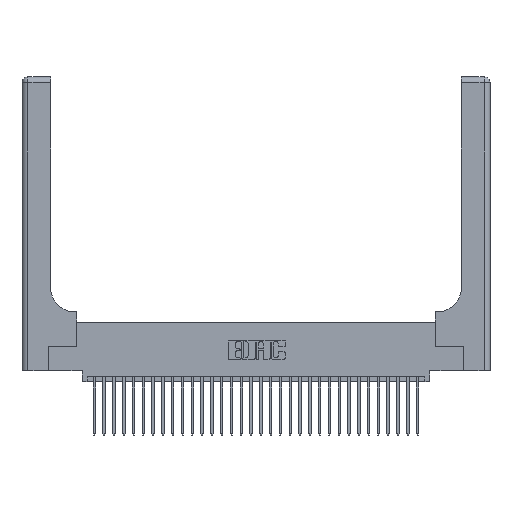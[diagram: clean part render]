
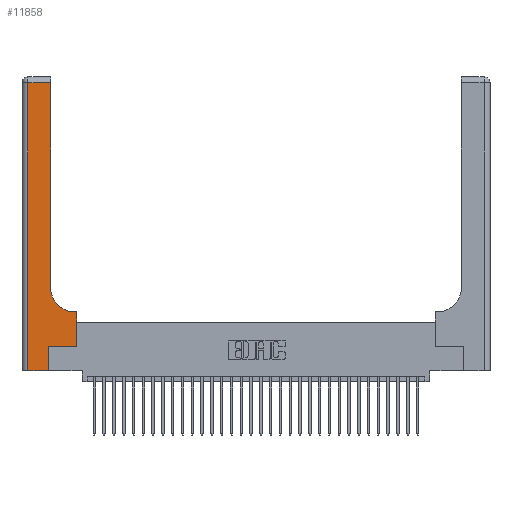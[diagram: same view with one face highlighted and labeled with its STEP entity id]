
A CAD part, top view. The second image highlights one B-rep face of the part: STEP entity #11858.
In plain terms, the highlighted planar face has unit normal (0, 0, 1).
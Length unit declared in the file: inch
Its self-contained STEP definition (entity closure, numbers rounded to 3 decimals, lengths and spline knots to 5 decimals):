
#128 = VECTOR ( 'NONE', #6298, 39.37008 ) ;
#644 = EDGE_CURVE ( 'NONE', #1270, #31202, #12621, .T. ) ;
#1270 = VERTEX_POINT ( 'NONE', #6350 ) ;
#1298 = DIRECTION ( 'NONE',  ( 0., 0., -1. ) ) ;
#2221 = VERTEX_POINT ( 'NONE', #28364 ) ;
#2227 = VERTEX_POINT ( 'NONE', #18069 ) ;
#2339 = EDGE_CURVE ( 'NONE', #2227, #22866, #31743, .T. ) ;
#2566 = EDGE_CURVE ( 'NONE', #31202, #2221, #10892, .T. ) ;
#2685 = EDGE_CURVE ( 'NONE', #2221, #3095, #14499, .T. ) ;
#3095 = VERTEX_POINT ( 'NONE', #18068 ) ;
#3262 = CARTESIAN_POINT ( 'NONE',  ( 0.5415, 0.85, 0.37 ) ) ;
#3271 = VECTOR ( 'NONE', #5865, 39.37008 ) ;
#3285 = CARTESIAN_POINT ( 'NONE',  ( 0.2915, 3., 0.37 ) ) ;
#3651 = LINE ( 'NONE', #20341, #30130 ) ;
#3737 = CARTESIAN_POINT ( 'NONE',  ( 0., 2.94, 0.37 ) ) ;
#3854 = ORIENTED_EDGE ( 'NONE', *, *, #2339, .T. ) ;
#5803 = EDGE_LOOP ( 'NONE', ( #15286, #8043, #31318, #31138, #18536, #3854, #11279, #20672, #7896 ) ) ;
#5838 = DIRECTION ( 'NONE',  ( 1., 0., 0. ) ) ;
#5865 = DIRECTION ( 'NONE',  ( 0., 1., 0. ) ) ;
#6298 = DIRECTION ( 'NONE',  ( -1., 0., 0. ) ) ;
#6350 = CARTESIAN_POINT ( 'NONE',  ( 0.5415, 0.6, 0.37 ) ) ;
#7566 = DIRECTION ( 'NONE',  ( 0., -1., 0. ) ) ;
#7896 = ORIENTED_EDGE ( 'NONE', *, *, #644, .T. ) ;
#8043 = ORIENTED_EDGE ( 'NONE', *, *, #2685, .T. ) ;
#8798 = CARTESIAN_POINT ( 'NONE',  ( 0.5585, 0.6, 0.37 ) ) ;
#9513 = CARTESIAN_POINT ( 'NONE',  ( 0.2915, 0.6, 0.37 ) ) ;
#10238 = EDGE_CURVE ( 'NONE', #3095, #19665, #3651, .T. ) ;
#10892 = LINE ( 'NONE', #3285, #3271 ) ;
#11007 = CARTESIAN_POINT ( 'NONE',  ( 0.269, 0., 0.37 ) ) ;
#11132 = FACE_OUTER_BOUND ( 'NONE', #5803, .T. ) ;
#11279 = ORIENTED_EDGE ( 'NONE', *, *, #28872, .T. ) ;
#11306 = VECTOR ( 'NONE', #16593, 39.37008 ) ;
#11858 = ADVANCED_FACE ( 'NONE', ( #11132 ), #31945, .F. ) ;
#12541 = CARTESIAN_POINT ( 'NONE',  ( 0.5585, 0.25, 0.37 ) ) ;
#12621 = CIRCLE ( 'NONE', #21081, 0.25 ) ;
#13258 = CARTESIAN_POINT ( 'NONE',  ( 0., 0., 0.37 ) ) ;
#13417 = VECTOR ( 'NONE', #18428, 39.37008 ) ;
#13473 = VECTOR ( 'NONE', #14662, 39.37008 ) ;
#14499 = LINE ( 'NONE', #3737, #128 ) ;
#14662 = DIRECTION ( 'NONE',  ( -1., 0., 0. ) ) ;
#14822 = EDGE_CURVE ( 'NONE', #22700, #1270, #33106, .T. ) ;
#15121 = DIRECTION ( 'NONE',  ( 0., 1., 0. ) ) ;
#15286 = ORIENTED_EDGE ( 'NONE', *, *, #2566, .T. ) ;
#15900 = VERTEX_POINT ( 'NONE', #31838 ) ;
#16593 = DIRECTION ( 'NONE',  ( 1., 0., 0. ) ) ;
#16603 = CARTESIAN_POINT ( 'NONE',  ( 0., 3., 0.37 ) ) ;
#17846 = VECTOR ( 'NONE', #18647, 39.37008 ) ;
#18068 = CARTESIAN_POINT ( 'NONE',  ( 0.06, 2.94, 0.37 ) ) ;
#18069 = CARTESIAN_POINT ( 'NONE',  ( 0.269, 0.25, 0.37 ) ) ;
#18428 = DIRECTION ( 'NONE',  ( 1., 0., 0. ) ) ;
#18536 = ORIENTED_EDGE ( 'NONE', *, *, #24691, .T. ) ;
#18647 = DIRECTION ( 'NONE',  ( 0., 1., 0. ) ) ;
#18840 = LINE ( 'NONE', #12541, #26444 ) ;
#19187 = DIRECTION ( 'NONE',  ( -1., 0., 0. ) ) ;
#19665 = VERTEX_POINT ( 'NONE', #21414 ) ;
#20235 = LINE ( 'NONE', #13258, #13417 ) ;
#20341 = CARTESIAN_POINT ( 'NONE',  ( 0.06, 3., 0.37 ) ) ;
#20672 = ORIENTED_EDGE ( 'NONE', *, *, #14822, .T. ) ;
#21081 = AXIS2_PLACEMENT_3D ( 'NONE', #3262, #21152, #5838 ) ;
#21152 = DIRECTION ( 'NONE',  ( 0., 0., -1. ) ) ;
#21414 = CARTESIAN_POINT ( 'NONE',  ( 0.06, 0., 0.37 ) ) ;
#22700 = VERTEX_POINT ( 'NONE', #8798 ) ;
#22866 = VERTEX_POINT ( 'NONE', #29878 ) ;
#24625 = EDGE_CURVE ( 'NONE', #19665, #15900, #20235, .T. ) ;
#24691 = EDGE_CURVE ( 'NONE', #15900, #2227, #31453, .T. ) ;
#24725 = AXIS2_PLACEMENT_3D ( 'NONE', #16603, #1298, #19187 ) ;
#26444 = VECTOR ( 'NONE', #15121, 39.37008 ) ;
#28364 = CARTESIAN_POINT ( 'NONE',  ( 0.2915, 2.94, 0.37 ) ) ;
#28872 = EDGE_CURVE ( 'NONE', #22866, #22700, #18840, .T. ) ;
#29857 = CARTESIAN_POINT ( 'NONE',  ( 0.2915, 0.85, 0.37 ) ) ;
#29878 = CARTESIAN_POINT ( 'NONE',  ( 0.5585, 0.25, 0.37 ) ) ;
#30130 = VECTOR ( 'NONE', #7566, 39.37008 ) ;
#31138 = ORIENTED_EDGE ( 'NONE', *, *, #24625, .T. ) ;
#31202 = VERTEX_POINT ( 'NONE', #29857 ) ;
#31318 = ORIENTED_EDGE ( 'NONE', *, *, #10238, .T. ) ;
#31453 = LINE ( 'NONE', #11007, #17846 ) ;
#31743 = LINE ( 'NONE', #31929, #11306 ) ;
#31838 = CARTESIAN_POINT ( 'NONE',  ( 0.269, 0., 0.37 ) ) ;
#31929 = CARTESIAN_POINT ( 'NONE',  ( 0.269, 0.25, 0.37 ) ) ;
#31945 = PLANE ( 'NONE',  #24725 ) ;
#33106 = LINE ( 'NONE', #9513, #13473 ) ;
